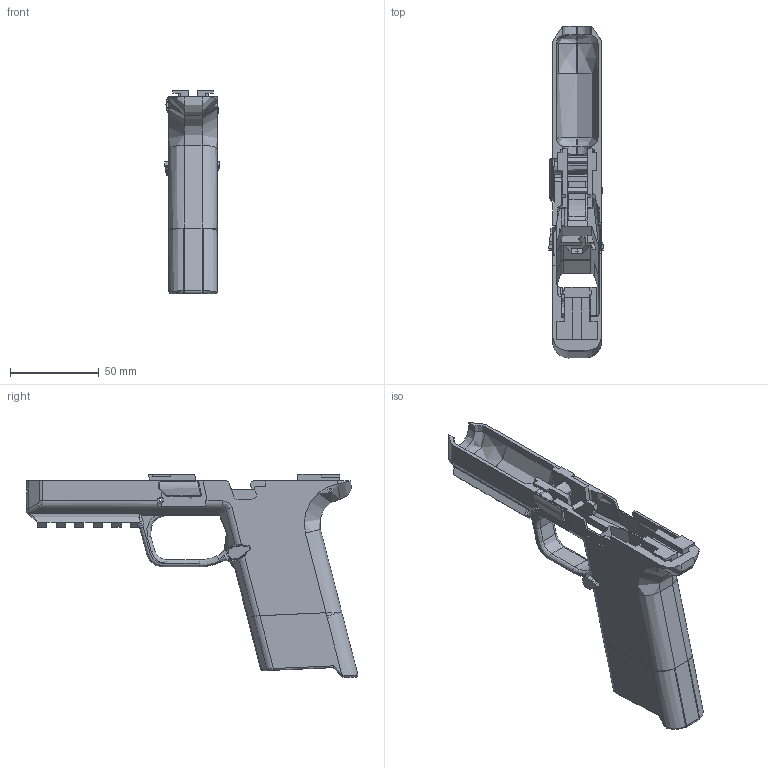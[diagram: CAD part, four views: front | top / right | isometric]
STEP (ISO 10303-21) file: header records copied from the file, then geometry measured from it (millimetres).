
FILE_DESCRIPTION(/* description */ (''),/* implementation_level */ '2;1');
FILE_NAME(/* name */ 'M&P 9 Assembly + Picatinny - Full Size Slide.step',/* time_stamp */ '2021-11-03T09:19:52-04:00',/* author */ (''),/* organization */ (''),/* preprocessor_version */ 'ST-DEVELOPER v18.1',/* originating_system */ 'Autodesk Translation Framework v10.10.0.1391',/* authorisation */ '');
FILE_SCHEMA (('AUTOMOTIVE_DESIGN { 1 0 10303 214 3 1 1 }'));
Length unit declared in the file: millimetre
Products named in the file (14): M&P 9 Standard Length Slide - Picatinny; M&P 9 Reference v99; Rear Fire Control Group Pin; Front Locking Block Group Pin; Trigger Pin; Locking Block; Disassembly Lug; Rear Fire Control Group; Frame; Trigger Guard and Magwell; Fitment Section; Nose; Magazine Release Button; Full-Size Magwell Body
Assembly tree (13 placements, depth 5):
  M&P 9 Standard Length Slide - Picatinny
    M&P 9 Reference v99
      Rear Fire Control Group Pin
      Front Locking Block Group Pin
      Trigger Pin
      Locking Block
      Disassembly Lug
      Rear Fire Control Group
      Frame
        Trigger Guard and Magwell
        Fitment Section
          Nose
        Magazine Release Button
        Full-Size Magwell Body
Bounding box: 30.85 x 187.13 x 114.63 mm (x, y, z)
Volume: 108392.7 mm3; surface area: 58807.5 mm2
Topology: 11 solids, 11 shells, 676 faces, 1846 edges, 1179 vertices
Faces by surface type: plane 365, cylinder 198, bspline 91, torus 17, sphere 4, cone 1
Full cylindrical faces by diameter (mm): 1.35 x2, 1.5 x3, 3.15 x2, 3.18 x3, 3.2 x2, 3.361 x2, 3.5 x1, 3.55 x4, 4.7 x2, 6.3 x1, 7.7 x1, 8.8 x1, 9 x2
Entity records: 24543 total; most frequent: CARTESIAN_POINT 7194, ORIENTED_EDGE 3684, DIRECTION 3393, EDGE_CURVE 1842, VERTEX_POINT 1179, LINE 1159, VECTOR 1159, AXIS2_PLACEMENT_3D 1117
